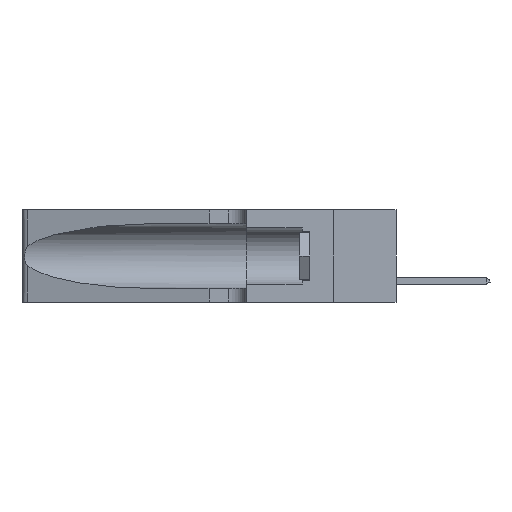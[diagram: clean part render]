
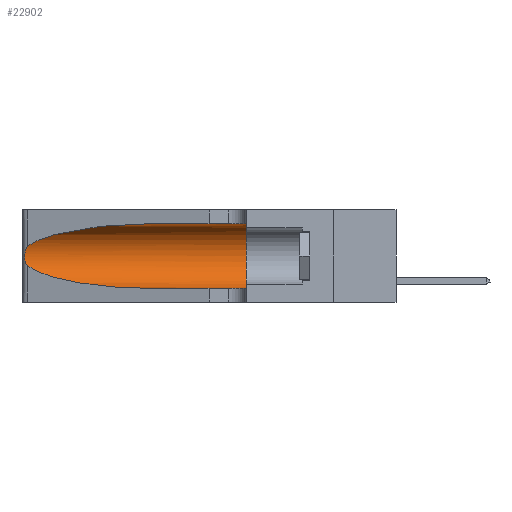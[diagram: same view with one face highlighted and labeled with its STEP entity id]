
A CAD part, left-side view. The second image highlights one B-rep face of the part: STEP entity #22902.
In plain terms, the highlighted cylindrical face has radius 3.308 mm (diameter 6.617 mm), a partial arc.
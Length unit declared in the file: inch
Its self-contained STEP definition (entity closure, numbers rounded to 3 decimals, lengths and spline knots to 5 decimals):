
#405 = ORIENTED_EDGE ( 'NONE', *, *, #15269, .T. ) ;
#511 = B_SPLINE_CURVE_WITH_KNOTS ( 'NONE', 3,
 ( #9017, #3169, #16661, #11047, #8751, #13021, #1399, #1223, #14894, #14978, #5242, #24288, #24375, #10709 ),
 .UNSPECIFIED., .F., .F.,
 ( 4, 2, 2, 2, 2, 2, 4 ),
 ( 0., 0.00027, 0.00053, 0.00107, 0.0016, 0.00187, 0.00214 ),
 .UNSPECIFIED. ) ;
#513 = FACE_OUTER_BOUND ( 'NONE', #7463, .T. ) ;
#675 = CARTESIAN_POINT ( 'NONE',  ( 0.1305, 1.61858, 0.05475 ) ) ;
#715 = EDGE_CURVE ( 'NONE', #14685, #6632, #2850, .T. ) ;
#888 = EDGE_CURVE ( 'NONE', #12116, #6632, #18633, .T. ) ;
#923 = CARTESIAN_POINT ( 'NONE',  ( 0.1305, 0.72297, 0.31525 ) ) ;
#1223 = CARTESIAN_POINT ( 'NONE',  ( 0.26075, 1.23896, 0.178 ) ) ;
#1399 = CARTESIAN_POINT ( 'NONE',  ( 0.26075, 1.23896, 0.19203 ) ) ;
#2850 = LINE ( 'NONE', #675, #17722 ) ;
#2855 = AXIS2_PLACEMENT_3D ( 'NONE', #5119, #14938, #20772 ) ;
#3112 = AXIS2_PLACEMENT_3D ( 'NONE', #10633, #16593, #20497 ) ;
#3169 = CARTESIAN_POINT ( 'NONE',  ( 0.25555, 1.22994, 0.2215 ) ) ;
#4543 = CARTESIAN_POINT ( 'NONE',  ( 0.18966, 0.96281, 0.31525 ) ) ;
#4993 =( BOUNDED_CURVE ( )  B_SPLINE_CURVE ( 3, ( #923, #4543, #22034, #16212 ),
 .UNSPECIFIED., .F., .T. ) 
 B_SPLINE_CURVE_WITH_KNOTS ( ( 4, 4 ),
 ( 1.5708, 2.84003 ),
 .UNSPECIFIED. ) 
 CURVE ( )  GEOMETRIC_REPRESENTATION_ITEM ( )  RATIONAL_B_SPLINE_CURVE ( ( 1., 0.87, 0.87, 1. ) ) 
 REPRESENTATION_ITEM ( '' )  );
#5119 = CARTESIAN_POINT ( 'NONE',  ( 0.1305, 0.35, 0.185 ) ) ;
#5242 = CARTESIAN_POINT ( 'NONE',  ( 0.25789, 1.23486, 0.15765 ) ) ;
#5585 = CARTESIAN_POINT ( 'NONE',  ( 0.18966, 0.96281, 0.05475 ) ) ;
#6632 = VERTEX_POINT ( 'NONE', #10358 ) ;
#6695 = CARTESIAN_POINT ( 'NONE',  ( 0.1305, 1.61858, 0.31525 ) ) ;
#7463 = EDGE_LOOP ( 'NONE', ( #24672, #405, #22344, #15403, #12926, #11400 ) ) ;
#8288 = DIRECTION ( 'NONE',  ( 0., -1., 0. ) ) ;
#8751 = CARTESIAN_POINT ( 'NONE',  ( 0.25854, 1.2359, 0.20912 ) ) ;
#9017 = CARTESIAN_POINT ( 'NONE',  ( 0.25487, 1.22718, 0.22369 ) ) ;
#9106 = CARTESIAN_POINT ( 'NONE',  ( 0.25487, 1.22718, 0.14631 ) ) ;
#10358 = CARTESIAN_POINT ( 'NONE',  ( 0.1305, 0.35, 0.05475 ) ) ;
#10633 = CARTESIAN_POINT ( 'NONE',  ( 0.1305, 1.61858, 0.185 ) ) ;
#10709 = CARTESIAN_POINT ( 'NONE',  ( 0.25487, 1.22718, 0.14631 ) ) ;
#11047 = CARTESIAN_POINT ( 'NONE',  ( 0.25787, 1.23484, 0.2124 ) ) ;
#11400 = ORIENTED_EDGE ( 'NONE', *, *, #17135, .F. ) ;
#11535 = VERTEX_POINT ( 'NONE', #15709 ) ;
#12116 = VERTEX_POINT ( 'NONE', #12396 ) ;
#12396 = CARTESIAN_POINT ( 'NONE',  ( 0.1305, 0.35, 0.31525 ) ) ;
#12926 = ORIENTED_EDGE ( 'NONE', *, *, #888, .F. ) ;
#13021 = CARTESIAN_POINT ( 'NONE',  ( 0.26018, 1.23835, 0.19895 ) ) ;
#13456 = CARTESIAN_POINT ( 'NONE',  ( 0.1305, 0.72297, 0.05475 ) ) ;
#13564 = CARTESIAN_POINT ( 'NONE',  ( 0.1305, 0.72297, 0.05475 ) ) ;
#14520 = VERTEX_POINT ( 'NONE', #15565 ) ;
#14685 = VERTEX_POINT ( 'NONE', #13564 ) ;
#14894 = CARTESIAN_POINT ( 'NONE',  ( 0.26017, 1.23833, 0.17102 ) ) ;
#14938 = DIRECTION ( 'NONE',  ( 0., 1., 0. ) ) ;
#14978 = CARTESIAN_POINT ( 'NONE',  ( 0.25856, 1.23593, 0.16098 ) ) ;
#15269 = EDGE_CURVE ( 'NONE', #21642, #11535, #511, .T. ) ;
#15285 = LINE ( 'NONE', #6695, #17079 ) ;
#15403 = ORIENTED_EDGE ( 'NONE', *, *, #715, .T. ) ;
#15565 = CARTESIAN_POINT ( 'NONE',  ( 0.1305, 0.72297, 0.31525 ) ) ;
#15709 = CARTESIAN_POINT ( 'NONE',  ( 0.25487, 1.22718, 0.14631 ) ) ;
#16212 = CARTESIAN_POINT ( 'NONE',  ( 0.25487, 1.22718, 0.22369 ) ) ;
#16593 = DIRECTION ( 'NONE',  ( 0., -1., 0. ) ) ;
#16661 = CARTESIAN_POINT ( 'NONE',  ( 0.25639, 1.23184, 0.21858 ) ) ;
#16825 = DIRECTION ( 'NONE',  ( 0., -1., 0. ) ) ;
#16987 = CARTESIAN_POINT ( 'NONE',  ( 0.2373, 1.15595, 0.08982 ) ) ;
#17079 = VECTOR ( 'NONE', #16825, 39.37008 ) ;
#17135 = EDGE_CURVE ( 'NONE', #14520, #12116, #15285, .T. ) ;
#17271 = EDGE_CURVE ( 'NONE', #11535, #14685, #20113, .T. ) ;
#17722 = VECTOR ( 'NONE', #8288, 39.37008 ) ;
#18633 = CIRCLE ( 'NONE', #2855, 0.13025 ) ;
#19149 = CARTESIAN_POINT ( 'NONE',  ( 0.25487, 1.22718, 0.22369 ) ) ;
#20113 =( BOUNDED_CURVE ( )  B_SPLINE_CURVE ( 3, ( #9106, #16987, #5585, #13456 ),
 .UNSPECIFIED., .F., .F. ) 
 B_SPLINE_CURVE_WITH_KNOTS ( ( 4, 4 ),
 ( 3.44316, 4.71239 ),
 .UNSPECIFIED. ) 
 CURVE ( )  GEOMETRIC_REPRESENTATION_ITEM ( )  RATIONAL_B_SPLINE_CURVE ( ( 1., 0.87, 0.87, 1. ) ) 
 REPRESENTATION_ITEM ( '' )  );
#20308 = EDGE_CURVE ( 'NONE', #14520, #21642, #4993, .T. ) ;
#20497 = DIRECTION ( 'NONE',  ( 0., 0., -1. ) ) ;
#20772 = DIRECTION ( 'NONE',  ( 0., 0., 1. ) ) ;
#21642 = VERTEX_POINT ( 'NONE', #19149 ) ;
#22034 = CARTESIAN_POINT ( 'NONE',  ( 0.2373, 1.15595, 0.28018 ) ) ;
#22344 = ORIENTED_EDGE ( 'NONE', *, *, #17271, .T. ) ;
#22902 = ADVANCED_FACE ( 'NONE', ( #513 ), #23585, .F. ) ;
#23585 = CYLINDRICAL_SURFACE ( 'NONE', #3112, 0.13025 ) ;
#24288 = CARTESIAN_POINT ( 'NONE',  ( 0.25639, 1.23186, 0.15144 ) ) ;
#24375 = CARTESIAN_POINT ( 'NONE',  ( 0.25555, 1.22993, 0.14849 ) ) ;
#24672 = ORIENTED_EDGE ( 'NONE', *, *, #20308, .T. ) ;
